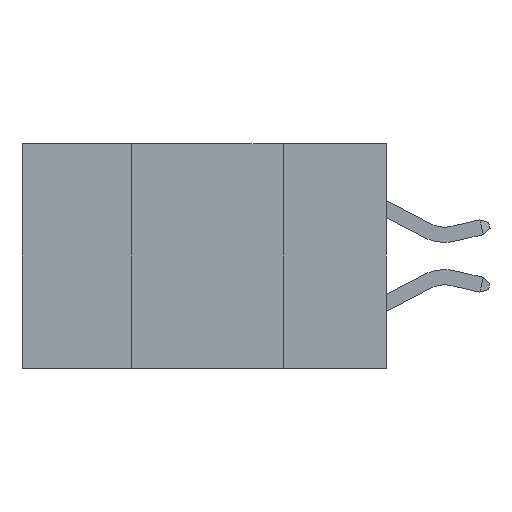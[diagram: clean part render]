
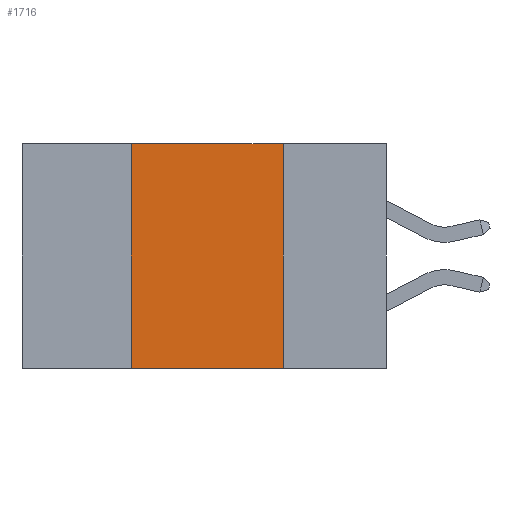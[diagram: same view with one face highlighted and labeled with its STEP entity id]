
A CAD part, left-side view. The second image highlights one B-rep face of the part: STEP entity #1716.
In plain terms, the highlighted planar face has unit normal (-1, 0, 0).
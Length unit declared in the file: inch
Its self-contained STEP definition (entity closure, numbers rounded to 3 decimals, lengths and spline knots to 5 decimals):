
#297 = CARTESIAN_POINT ( 'NONE',  ( 0., 0.6, 0. ) ) ;
#1124 = AXIS2_PLACEMENT_3D ( 'NONE', #14983, #13463, #13193 ) ;
#1537 = CARTESIAN_POINT ( 'NONE',  ( 0., 0.17, 0. ) ) ;
#1609 = CARTESIAN_POINT ( 'NONE',  ( 0., 0.17, 0. ) ) ;
#1716 = ADVANCED_FACE ( 'NONE', ( #23144 ), #14927, .F. ) ;
#1793 = ORIENTED_EDGE ( 'NONE', *, *, #11559, .F. ) ;
#2642 = VERTEX_POINT ( 'NONE', #19957 ) ;
#3404 = EDGE_CURVE ( 'NONE', #16014, #2642, #10269, .T. ) ;
#3479 = VECTOR ( 'NONE', #15228, 39.37008 ) ;
#3932 = CARTESIAN_POINT ( 'NONE',  ( 0., 0.6, -0.37 ) ) ;
#5267 = VECTOR ( 'NONE', #21715, 39.37008 ) ;
#5750 = ORIENTED_EDGE ( 'NONE', *, *, #14687, .F. ) ;
#5851 = DIRECTION ( 'NONE',  ( 0., -1., 0. ) ) ;
#6558 = CARTESIAN_POINT ( 'NONE',  ( 0., 0.42, 0. ) ) ;
#7101 = ORIENTED_EDGE ( 'NONE', *, *, #18301, .T. ) ;
#8219 = LINE ( 'NONE', #3932, #17427 ) ;
#10269 = LINE ( 'NONE', #6558, #5267 ) ;
#11559 = EDGE_CURVE ( 'NONE', #2642, #16532, #18258, .T. ) ;
#12778 = DIRECTION ( 'NONE',  ( 0., 0., -1. ) ) ;
#13193 = DIRECTION ( 'NONE',  ( 0., 0., -1. ) ) ;
#13463 = DIRECTION ( 'NONE',  ( 1., 0., 0. ) ) ;
#13674 = LINE ( 'NONE', #1537, #17914 ) ;
#14687 = EDGE_CURVE ( 'NONE', #16532, #17020, #13674, .T. ) ;
#14927 = PLANE ( 'NONE',  #1124 ) ;
#14983 = CARTESIAN_POINT ( 'NONE',  ( 0., 0.6, 0. ) ) ;
#15228 = DIRECTION ( 'NONE',  ( 0., -1., 0. ) ) ;
#16014 = VERTEX_POINT ( 'NONE', #22198 ) ;
#16245 = CARTESIAN_POINT ( 'NONE',  ( 0., 0.17, -0.37 ) ) ;
#16532 = VERTEX_POINT ( 'NONE', #1609 ) ;
#17020 = VERTEX_POINT ( 'NONE', #16245 ) ;
#17427 = VECTOR ( 'NONE', #5851, 39.37008 ) ;
#17914 = VECTOR ( 'NONE', #12778, 39.37008 ) ;
#18258 = LINE ( 'NONE', #297, #3479 ) ;
#18301 = EDGE_CURVE ( 'NONE', #16014, #17020, #8219, .T. ) ;
#19939 = ORIENTED_EDGE ( 'NONE', *, *, #3404, .F. ) ;
#19957 = CARTESIAN_POINT ( 'NONE',  ( 0., 0.42, 0. ) ) ;
#21715 = DIRECTION ( 'NONE',  ( 0., 0., 1. ) ) ;
#21813 = EDGE_LOOP ( 'NONE', ( #5750, #1793, #19939, #7101 ) ) ;
#22198 = CARTESIAN_POINT ( 'NONE',  ( 0., 0.42, -0.37 ) ) ;
#23144 = FACE_OUTER_BOUND ( 'NONE', #21813, .T. ) ;
